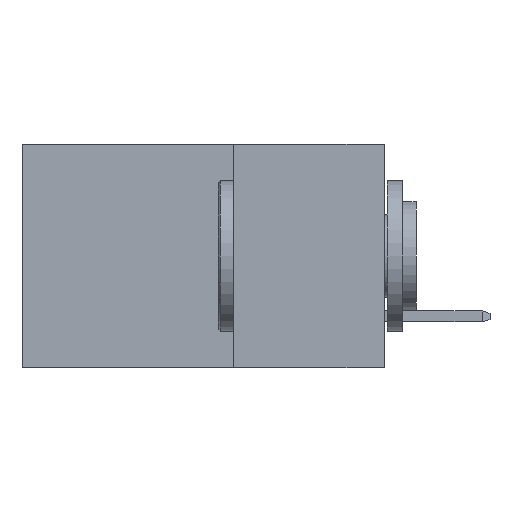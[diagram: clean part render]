
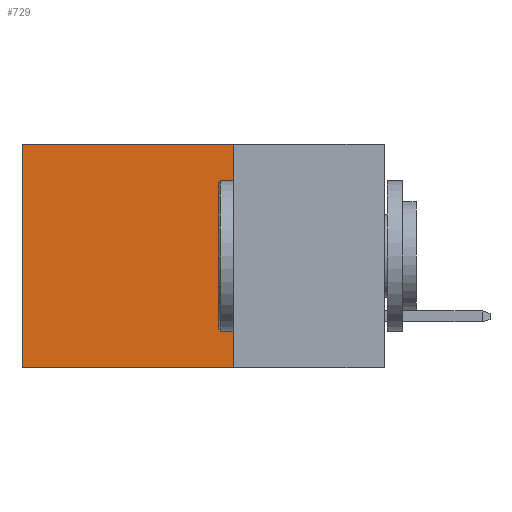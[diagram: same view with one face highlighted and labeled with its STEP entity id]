
A CAD part, left-side view. The second image highlights one B-rep face of the part: STEP entity #729.
In plain terms, the highlighted planar face has unit normal (-1, 0, 0).
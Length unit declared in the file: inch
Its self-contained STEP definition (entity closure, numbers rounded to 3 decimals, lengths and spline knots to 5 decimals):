
#218 = LINE ( 'NONE', #4802, #4557 ) ;
#488 = CARTESIAN_POINT ( 'NONE',  ( 0.298, 0.6, 0. ) ) ;
#729 = ADVANCED_FACE ( 'NONE', ( #6823 ), #4834, .F. ) ;
#1075 = CARTESIAN_POINT ( 'NONE',  ( 0.298, 0.25, 0. ) ) ;
#1446 = VECTOR ( 'NONE', #10429, 39.37008 ) ;
#1506 = AXIS2_PLACEMENT_3D ( 'NONE', #4885, #4832, #4808 ) ;
#1624 = VECTOR ( 'NONE', #4603, 39.37008 ) ;
#1951 = EDGE_CURVE ( 'NONE', #3404, #3098, #6067, .T. ) ;
#1980 = EDGE_CURVE ( 'NONE', #10767, #3098, #10290, .T. ) ;
#2920 = EDGE_LOOP ( 'NONE', ( #9496, #4782, #6080, #8110 ) ) ;
#3098 = VERTEX_POINT ( 'NONE', #9968 ) ;
#3404 = VERTEX_POINT ( 'NONE', #9909 ) ;
#3618 = VERTEX_POINT ( 'NONE', #9773 ) ;
#4557 = VECTOR ( 'NONE', #9135, 39.37008 ) ;
#4603 = DIRECTION ( 'NONE',  ( 0., 0., -1. ) ) ;
#4782 = ORIENTED_EDGE ( 'NONE', *, *, #1951, .F. ) ;
#4802 = CARTESIAN_POINT ( 'NONE',  ( 0.298, 0.25, 0. ) ) ;
#4808 = DIRECTION ( 'NONE',  ( 0., 0., -1. ) ) ;
#4832 = DIRECTION ( 'NONE',  ( 1., 0., 0. ) ) ;
#4834 = PLANE ( 'NONE',  #1506 ) ;
#4885 = CARTESIAN_POINT ( 'NONE',  ( 0.298, 0.25, 0. ) ) ;
#5519 = VECTOR ( 'NONE', #5615, 39.37008 ) ;
#5615 = DIRECTION ( 'NONE',  ( 0., 0., -1. ) ) ;
#6067 = LINE ( 'NONE', #10529, #1446 ) ;
#6080 = ORIENTED_EDGE ( 'NONE', *, *, #6653, .F. ) ;
#6531 = CARTESIAN_POINT ( 'NONE',  ( 0.298, 0.6, 0. ) ) ;
#6653 = EDGE_CURVE ( 'NONE', #3618, #3404, #8560, .T. ) ;
#6823 = FACE_OUTER_BOUND ( 'NONE', #2920, .T. ) ;
#8110 = ORIENTED_EDGE ( 'NONE', *, *, #8976, .T. ) ;
#8560 = LINE ( 'NONE', #1075, #1624 ) ;
#8976 = EDGE_CURVE ( 'NONE', #3618, #10767, #218, .T. ) ;
#9135 = DIRECTION ( 'NONE',  ( 0., 1., 0. ) ) ;
#9496 = ORIENTED_EDGE ( 'NONE', *, *, #1980, .T. ) ;
#9773 = CARTESIAN_POINT ( 'NONE',  ( 0.298, 0.25, 0. ) ) ;
#9909 = CARTESIAN_POINT ( 'NONE',  ( 0.298, 0.25, -0.37 ) ) ;
#9968 = CARTESIAN_POINT ( 'NONE',  ( 0.298, 0.6, -0.37 ) ) ;
#10290 = LINE ( 'NONE', #6531, #5519 ) ;
#10429 = DIRECTION ( 'NONE',  ( 0., 1., 0. ) ) ;
#10529 = CARTESIAN_POINT ( 'NONE',  ( 0.298, 0.25, -0.37 ) ) ;
#10767 = VERTEX_POINT ( 'NONE', #488 ) ;
